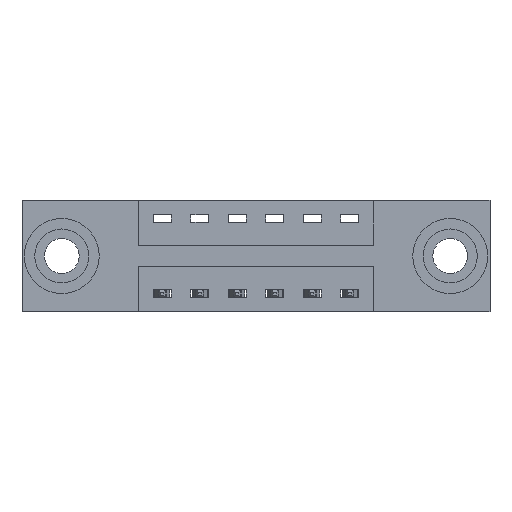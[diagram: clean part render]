
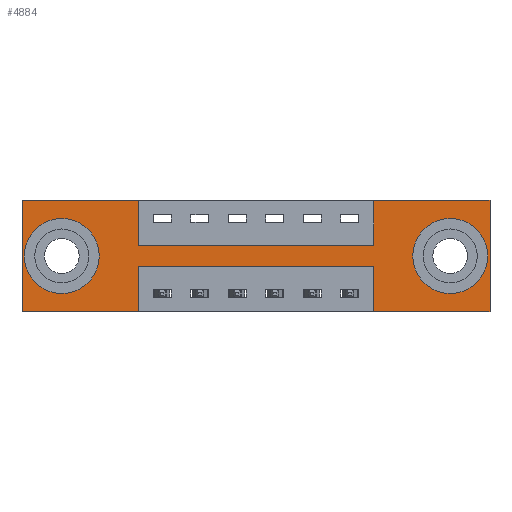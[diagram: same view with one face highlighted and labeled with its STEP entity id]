
A CAD part, front view. The second image highlights one B-rep face of the part: STEP entity #4884.
In plain terms, the highlighted planar face has unit normal (0, -1, 0).
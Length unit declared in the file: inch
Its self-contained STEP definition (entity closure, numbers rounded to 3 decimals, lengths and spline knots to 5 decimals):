
#63 = ORIENTED_EDGE ( 'NONE', *, *, #4342, .F. ) ;
#247 = VECTOR ( 'NONE', #1827, 39.37008 ) ;
#310 = VECTOR ( 'NONE', #8165, 39.37008 ) ;
#629 = VERTEX_POINT ( 'NONE', #3377 ) ;
#702 = CARTESIAN_POINT ( 'NONE',  ( 0., 0., 0. ) ) ;
#839 = LINE ( 'NONE', #4577, #1068 ) ;
#863 = CARTESIAN_POINT ( 'NONE',  ( 0.3875, 0., -0.22 ) ) ;
#892 = VERTEX_POINT ( 'NONE', #1200 ) ;
#904 = EDGE_CURVE ( 'NONE', #3473, #6416, #3204, .T. ) ;
#919 = EDGE_CURVE ( 'NONE', #892, #6925, #9012, .T. ) ;
#958 = ORIENTED_EDGE ( 'NONE', *, *, #1083, .F. ) ;
#964 = DIRECTION ( 'NONE',  ( -1., 0., 0. ) ) ;
#1004 = EDGE_LOOP ( 'NONE', ( #8806, #63, #7449, #1086, #1272, #3585, #1555, #7608, #1798, #9164, #3451, #958 ) ) ;
#1024 = DIRECTION ( 'NONE',  ( 0., 0., 1. ) ) ;
#1068 = VECTOR ( 'NONE', #3061, 39.37008 ) ;
#1083 = EDGE_CURVE ( 'NONE', #7041, #629, #2321, .T. ) ;
#1086 = ORIENTED_EDGE ( 'NONE', *, *, #3068, .F. ) ;
#1173 = EDGE_CURVE ( 'NONE', #4199, #7949, #6314, .T. ) ;
#1200 = CARTESIAN_POINT ( 'NONE',  ( 1.4275, 0., -0.107 ) ) ;
#1272 = ORIENTED_EDGE ( 'NONE', *, *, #8599, .F. ) ;
#1459 = VERTEX_POINT ( 'NONE', #5068 ) ;
#1469 = ORIENTED_EDGE ( 'NONE', *, *, #5084, .T. ) ;
#1555 = ORIENTED_EDGE ( 'NONE', *, *, #5162, .F. ) ;
#1569 = DIRECTION ( 'NONE',  ( 0., -1., 0. ) ) ;
#1661 = AXIS2_PLACEMENT_3D ( 'NONE', #7772, #5645, #8654 ) ;
#1667 = CARTESIAN_POINT ( 'NONE',  ( 1.56, 0., 0. ) ) ;
#1701 = AXIS2_PLACEMENT_3D ( 'NONE', #3071, #1569, #1769 ) ;
#1739 = ORIENTED_EDGE ( 'NONE', *, *, #8494, .T. ) ;
#1769 = DIRECTION ( 'NONE',  ( 0., 0., -1. ) ) ;
#1798 = ORIENTED_EDGE ( 'NONE', *, *, #6000, .F. ) ;
#1827 = DIRECTION ( 'NONE',  ( -1., 0., 0. ) ) ;
#2008 = VECTOR ( 'NONE', #964, 39.37008 ) ;
#2132 = LINE ( 'NONE', #6867, #5959 ) ;
#2151 = CARTESIAN_POINT ( 'NONE',  ( 0.3875, 0., -0.15 ) ) ;
#2156 = EDGE_CURVE ( 'NONE', #4625, #5905, #839, .T. ) ;
#2174 = CARTESIAN_POINT ( 'NONE',  ( 1.56, 0., 0. ) ) ;
#2321 = LINE ( 'NONE', #2470, #4778 ) ;
#2406 = FACE_BOUND ( 'NONE', #7827, .T. ) ;
#2470 = CARTESIAN_POINT ( 'NONE',  ( 0., 0., -0.37 ) ) ;
#2678 = DIRECTION ( 'NONE',  ( 0., 1., 0. ) ) ;
#2712 = EDGE_CURVE ( 'NONE', #6891, #7041, #6257, .T. ) ;
#2747 = LINE ( 'NONE', #702, #6742 ) ;
#2834 = CARTESIAN_POINT ( 'NONE',  ( 0.1325, 0., -0.185 ) ) ;
#2917 = VECTOR ( 'NONE', #5578, 39.37008 ) ;
#2955 = CARTESIAN_POINT ( 'NONE',  ( 0.3875, 0., 0. ) ) ;
#3061 = DIRECTION ( 'NONE',  ( 1., 0., 0. ) ) ;
#3068 = EDGE_CURVE ( 'NONE', #1459, #4199, #5548, .T. ) ;
#3071 = CARTESIAN_POINT ( 'NONE',  ( 0., 0., -0.37 ) ) ;
#3178 = CARTESIAN_POINT ( 'NONE',  ( 0.1325, 0., -0.263 ) ) ;
#3195 = CARTESIAN_POINT ( 'NONE',  ( 1.1725, 0., 0. ) ) ;
#3204 = CIRCLE ( 'NONE', #6338, 0.078 ) ;
#3227 = CARTESIAN_POINT ( 'NONE',  ( 0., 0., -0.37 ) ) ;
#3377 = CARTESIAN_POINT ( 'NONE',  ( 0., 0., -0.37 ) ) ;
#3402 = VECTOR ( 'NONE', #5609, 39.37008 ) ;
#3451 = ORIENTED_EDGE ( 'NONE', *, *, #5291, .F. ) ;
#3473 = VERTEX_POINT ( 'NONE', #4066 ) ;
#3499 = LINE ( 'NONE', #2174, #310 ) ;
#3585 = ORIENTED_EDGE ( 'NONE', *, *, #8827, .F. ) ;
#3706 = DIRECTION ( 'NONE',  ( 0., 0., -1. ) ) ;
#3786 = ORIENTED_EDGE ( 'NONE', *, *, #904, .T. ) ;
#3881 = CIRCLE ( 'NONE', #5165, 0.078 ) ;
#4066 = CARTESIAN_POINT ( 'NONE',  ( 0.1325, 0., -0.107 ) ) ;
#4199 = VERTEX_POINT ( 'NONE', #4303 ) ;
#4200 = CARTESIAN_POINT ( 'NONE',  ( 0.1325, 0., -0.185 ) ) ;
#4303 = CARTESIAN_POINT ( 'NONE',  ( 1.1725, 0., -0.37 ) ) ;
#4342 = EDGE_CURVE ( 'NONE', #7949, #6891, #6858, .T. ) ;
#4437 = CARTESIAN_POINT ( 'NONE',  ( 1.4275, 0., -0.185 ) ) ;
#4577 = CARTESIAN_POINT ( 'NONE',  ( 0.3875, 0., -0.15 ) ) ;
#4590 = FACE_OUTER_BOUND ( 'NONE', #1004, .T. ) ;
#4625 = VERTEX_POINT ( 'NONE', #2151 ) ;
#4627 = CARTESIAN_POINT ( 'NONE',  ( 1.1725, 0., 0. ) ) ;
#4778 = VECTOR ( 'NONE', #8967, 39.37008 ) ;
#4884 = ADVANCED_FACE ( 'NONE', ( #7556, #2406, #4590 ), #8332, .T. ) ;
#4959 = LINE ( 'NONE', #7089, #3402 ) ;
#4972 = VECTOR ( 'NONE', #1024, 39.37008 ) ;
#5022 = CARTESIAN_POINT ( 'NONE',  ( 1.4275, 0., -0.263 ) ) ;
#5068 = CARTESIAN_POINT ( 'NONE',  ( 1.56, 0., -0.37 ) ) ;
#5069 = CARTESIAN_POINT ( 'NONE',  ( 0.3875, 0., -0.37 ) ) ;
#5084 = EDGE_CURVE ( 'NONE', #6416, #3473, #8131, .T. ) ;
#5148 = VECTOR ( 'NONE', #3706, 39.37008 ) ;
#5162 = EDGE_CURVE ( 'NONE', #5905, #5223, #8986, .T. ) ;
#5165 = AXIS2_PLACEMENT_3D ( 'NONE', #4437, #7437, #6694 ) ;
#5223 = VERTEX_POINT ( 'NONE', #3195 ) ;
#5291 = EDGE_CURVE ( 'NONE', #629, #5775, #4959, .T. ) ;
#5501 = CARTESIAN_POINT ( 'NONE',  ( 0., 0., 0. ) ) ;
#5545 = DIRECTION ( 'NONE',  ( 0., 0., 1. ) ) ;
#5548 = LINE ( 'NONE', #3227, #247 ) ;
#5578 = DIRECTION ( 'NONE',  ( 0., 0., -1. ) ) ;
#5609 = DIRECTION ( 'NONE',  ( 0., 0., 1. ) ) ;
#5645 = DIRECTION ( 'NONE',  ( 0., 1., 0. ) ) ;
#5722 = CARTESIAN_POINT ( 'NONE',  ( 0.3875, 0., -0.22 ) ) ;
#5775 = VERTEX_POINT ( 'NONE', #5501 ) ;
#5781 = CARTESIAN_POINT ( 'NONE',  ( 1.1725, 0., -0.15 ) ) ;
#5905 = VERTEX_POINT ( 'NONE', #5781 ) ;
#5959 = VECTOR ( 'NONE', #9169, 39.37008 ) ;
#6000 = EDGE_CURVE ( 'NONE', #9269, #4625, #6022, .T. ) ;
#6022 = LINE ( 'NONE', #2955, #5148 ) ;
#6123 = VERTEX_POINT ( 'NONE', #1667 ) ;
#6257 = LINE ( 'NONE', #9249, #2917 ) ;
#6314 = LINE ( 'NONE', #7761, #7284 ) ;
#6338 = AXIS2_PLACEMENT_3D ( 'NONE', #4200, #2678, #7216 ) ;
#6416 = VERTEX_POINT ( 'NONE', #3178 ) ;
#6694 = DIRECTION ( 'NONE',  ( 0., 0., -1. ) ) ;
#6742 = VECTOR ( 'NONE', #7252, 39.37008 ) ;
#6858 = LINE ( 'NONE', #863, #2008 ) ;
#6867 = CARTESIAN_POINT ( 'NONE',  ( 0., 0., 0. ) ) ;
#6891 = VERTEX_POINT ( 'NONE', #5722 ) ;
#6925 = VERTEX_POINT ( 'NONE', #5022 ) ;
#7041 = VERTEX_POINT ( 'NONE', #5069 ) ;
#7089 = CARTESIAN_POINT ( 'NONE',  ( 0., 0., 0. ) ) ;
#7216 = DIRECTION ( 'NONE',  ( 0., 0., 1. ) ) ;
#7252 = DIRECTION ( 'NONE',  ( 1., 0., 0. ) ) ;
#7284 = VECTOR ( 'NONE', #5545, 39.37008 ) ;
#7389 = EDGE_LOOP ( 'NONE', ( #9602, #1739 ) ) ;
#7436 = DIRECTION ( 'NONE',  ( 0., 0., 1. ) ) ;
#7437 = DIRECTION ( 'NONE',  ( 0., 1., 0. ) ) ;
#7449 = ORIENTED_EDGE ( 'NONE', *, *, #1173, .F. ) ;
#7556 = FACE_BOUND ( 'NONE', #7389, .T. ) ;
#7608 = ORIENTED_EDGE ( 'NONE', *, *, #2156, .F. ) ;
#7752 = EDGE_CURVE ( 'NONE', #5775, #9269, #2132, .T. ) ;
#7761 = CARTESIAN_POINT ( 'NONE',  ( 1.1725, 0., -0.37 ) ) ;
#7772 = CARTESIAN_POINT ( 'NONE',  ( 1.4275, 0., -0.185 ) ) ;
#7827 = EDGE_LOOP ( 'NONE', ( #3786, #1469 ) ) ;
#7949 = VERTEX_POINT ( 'NONE', #9554 ) ;
#8131 = CIRCLE ( 'NONE', #9206, 0.078 ) ;
#8165 = DIRECTION ( 'NONE',  ( 0., 0., -1. ) ) ;
#8332 = PLANE ( 'NONE',  #1701 ) ;
#8420 = CARTESIAN_POINT ( 'NONE',  ( 0.3875, 0., 0. ) ) ;
#8494 = EDGE_CURVE ( 'NONE', #6925, #892, #3881, .T. ) ;
#8599 = EDGE_CURVE ( 'NONE', #6123, #1459, #3499, .T. ) ;
#8654 = DIRECTION ( 'NONE',  ( 0., 0., -1. ) ) ;
#8806 = ORIENTED_EDGE ( 'NONE', *, *, #2712, .F. ) ;
#8827 = EDGE_CURVE ( 'NONE', #5223, #6123, #2747, .T. ) ;
#8967 = DIRECTION ( 'NONE',  ( -1., 0., 0. ) ) ;
#8986 = LINE ( 'NONE', #4627, #4972 ) ;
#9012 = CIRCLE ( 'NONE', #1661, 0.078 ) ;
#9164 = ORIENTED_EDGE ( 'NONE', *, *, #7752, .F. ) ;
#9169 = DIRECTION ( 'NONE',  ( 1., 0., 0. ) ) ;
#9206 = AXIS2_PLACEMENT_3D ( 'NONE', #2834, #9526, #7436 ) ;
#9249 = CARTESIAN_POINT ( 'NONE',  ( 0.3875, 0., -0.37 ) ) ;
#9269 = VERTEX_POINT ( 'NONE', #8420 ) ;
#9526 = DIRECTION ( 'NONE',  ( 0., 1., 0. ) ) ;
#9554 = CARTESIAN_POINT ( 'NONE',  ( 1.1725, 0., -0.22 ) ) ;
#9602 = ORIENTED_EDGE ( 'NONE', *, *, #919, .T. ) ;
